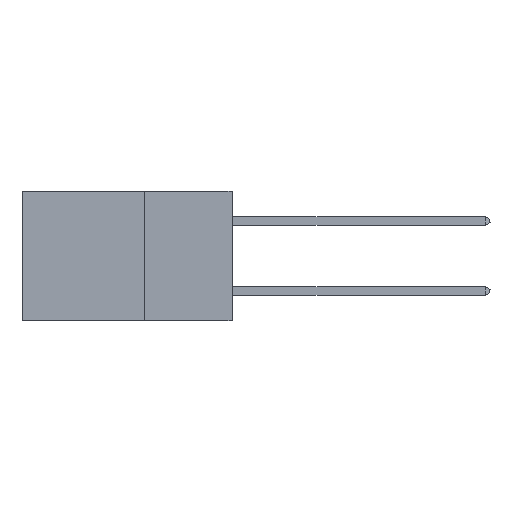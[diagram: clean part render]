
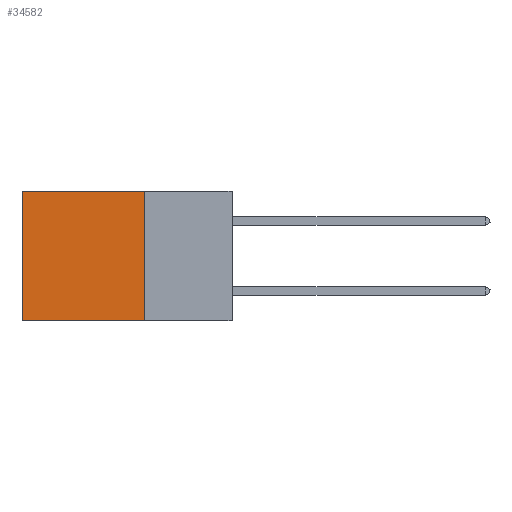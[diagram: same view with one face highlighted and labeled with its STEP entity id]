
A CAD part, left-side view. The second image highlights one B-rep face of the part: STEP entity #34582.
In plain terms, the highlighted planar face has unit normal (-1, 0, 0).
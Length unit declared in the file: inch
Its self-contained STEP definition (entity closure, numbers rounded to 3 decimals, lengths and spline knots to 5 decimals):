
#621 = CARTESIAN_POINT ( 'NONE',  ( 0.2875, 0.6, 0. ) ) ;
#1101 = DIRECTION ( 'NONE',  ( 0., 0., -1. ) ) ;
#1640 = EDGE_LOOP ( 'NONE', ( #8328, #31166, #25207, #35539 ) ) ;
#2266 = CARTESIAN_POINT ( 'NONE',  ( 0.2875, 0.25, 0. ) ) ;
#2476 = DIRECTION ( 'NONE',  ( 0., 0., -1. ) ) ;
#3107 = CARTESIAN_POINT ( 'NONE',  ( 0.2875, 0.25, 0. ) ) ;
#3340 = VERTEX_POINT ( 'NONE', #32759 ) ;
#5069 = CARTESIAN_POINT ( 'NONE',  ( 0.2875, 0.25, 0. ) ) ;
#6882 = FACE_OUTER_BOUND ( 'NONE', #1640, .T. ) ;
#7382 = VERTEX_POINT ( 'NONE', #13532 ) ;
#8328 = ORIENTED_EDGE ( 'NONE', *, *, #21049, .T. ) ;
#9166 = VECTOR ( 'NONE', #2476, 39.37008 ) ;
#10938 = LINE ( 'NONE', #19197, #9166 ) ;
#11946 = VERTEX_POINT ( 'NONE', #13023 ) ;
#12099 = VECTOR ( 'NONE', #1101, 39.37008 ) ;
#12563 = LINE ( 'NONE', #621, #12099 ) ;
#12985 = DIRECTION ( 'NONE',  ( 0., 1., 0. ) ) ;
#13023 = CARTESIAN_POINT ( 'NONE',  ( 0.2875, 0.25, -0.37 ) ) ;
#13532 = CARTESIAN_POINT ( 'NONE',  ( 0.2875, 0.6, -0.37 ) ) ;
#19197 = CARTESIAN_POINT ( 'NONE',  ( 0.2875, 0.25, 0. ) ) ;
#19818 = EDGE_CURVE ( 'NONE', #11946, #7382, #32722, .T. ) ;
#20011 = VERTEX_POINT ( 'NONE', #2266 ) ;
#20318 = AXIS2_PLACEMENT_3D ( 'NONE', #3107, #25644, #28454 ) ;
#21049 = EDGE_CURVE ( 'NONE', #3340, #7382, #12563, .T. ) ;
#21288 = DIRECTION ( 'NONE',  ( 0., 1., 0. ) ) ;
#22186 = EDGE_CURVE ( 'NONE', #20011, #3340, #26926, .T. ) ;
#24934 = EDGE_CURVE ( 'NONE', #20011, #11946, #10938, .T. ) ;
#25207 = ORIENTED_EDGE ( 'NONE', *, *, #24934, .F. ) ;
#25409 = PLANE ( 'NONE',  #20318 ) ;
#25644 = DIRECTION ( 'NONE',  ( 1., 0., 0. ) ) ;
#26926 = LINE ( 'NONE', #5069, #33850 ) ;
#28454 = DIRECTION ( 'NONE',  ( 0., 0., -1. ) ) ;
#29261 = VECTOR ( 'NONE', #12985, 39.37008 ) ;
#31166 = ORIENTED_EDGE ( 'NONE', *, *, #19818, .F. ) ;
#32377 = CARTESIAN_POINT ( 'NONE',  ( 0.2875, 0.25, -0.37 ) ) ;
#32722 = LINE ( 'NONE', #32377, #29261 ) ;
#32759 = CARTESIAN_POINT ( 'NONE',  ( 0.2875, 0.6, 0. ) ) ;
#33850 = VECTOR ( 'NONE', #21288, 39.37008 ) ;
#34582 = ADVANCED_FACE ( 'NONE', ( #6882 ), #25409, .F. ) ;
#35539 = ORIENTED_EDGE ( 'NONE', *, *, #22186, .T. ) ;
